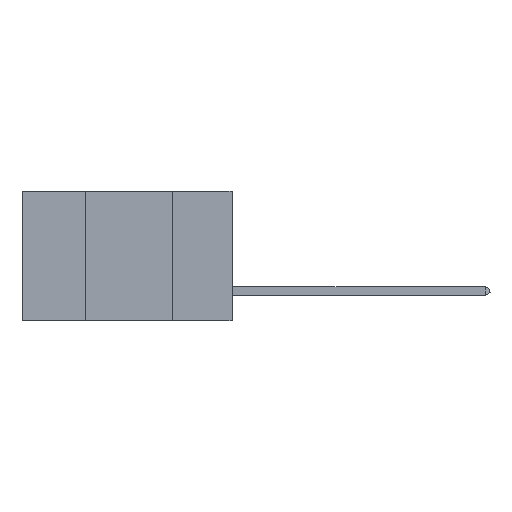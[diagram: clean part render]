
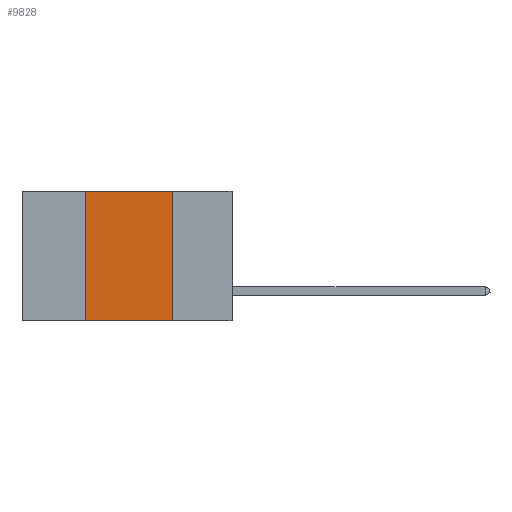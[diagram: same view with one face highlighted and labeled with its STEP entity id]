
A CAD part, left-side view. The second image highlights one B-rep face of the part: STEP entity #9828.
In plain terms, the highlighted planar face has unit normal (-1, 0, 0).
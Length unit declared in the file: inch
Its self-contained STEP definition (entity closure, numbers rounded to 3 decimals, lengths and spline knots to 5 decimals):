
#146 = CARTESIAN_POINT ( 'NONE',  ( 0., 0.42, -0.37 ) ) ;
#923 = CARTESIAN_POINT ( 'NONE',  ( 0., 0.17, 0. ) ) ;
#2415 = EDGE_CURVE ( 'NONE', #5832, #20994, #16432, .T. ) ;
#2769 = ORIENTED_EDGE ( 'NONE', *, *, #3607, .F. ) ;
#3252 = CARTESIAN_POINT ( 'NONE',  ( 0., 0.6, -0.37 ) ) ;
#3427 = CARTESIAN_POINT ( 'NONE',  ( 0., 0.6, 0. ) ) ;
#3607 = EDGE_CURVE ( 'NONE', #13845, #20994, #19619, .T. ) ;
#5685 = VECTOR ( 'NONE', #18300, 39.37008 ) ;
#5832 = VERTEX_POINT ( 'NONE', #146 ) ;
#5968 = VECTOR ( 'NONE', #15742, 39.37008 ) ;
#6342 = EDGE_CURVE ( 'NONE', #8032, #13845, #15232, .T. ) ;
#6881 = DIRECTION ( 'NONE',  ( 0., 0., -1. ) ) ;
#7025 = DIRECTION ( 'NONE',  ( 0., 0., 1. ) ) ;
#8032 = VERTEX_POINT ( 'NONE', #15239 ) ;
#8890 = EDGE_CURVE ( 'NONE', #5832, #8032, #10215, .T. ) ;
#8909 = CARTESIAN_POINT ( 'NONE',  ( 0., 0.17, -0.37 ) ) ;
#8925 = PLANE ( 'NONE',  #9853 ) ;
#9828 = ADVANCED_FACE ( 'NONE', ( #15352 ), #8925, .F. ) ;
#9853 = AXIS2_PLACEMENT_3D ( 'NONE', #3427, #18009, #6881 ) ;
#10215 = LINE ( 'NONE', #23651, #16572 ) ;
#12585 = VECTOR ( 'NONE', #15078, 39.37008 ) ;
#12643 = CARTESIAN_POINT ( 'NONE',  ( 0., 0.6, 0. ) ) ;
#12980 = ORIENTED_EDGE ( 'NONE', *, *, #8890, .F. ) ;
#13845 = VERTEX_POINT ( 'NONE', #923 ) ;
#15078 = DIRECTION ( 'NONE',  ( 0., 0., -1. ) ) ;
#15232 = LINE ( 'NONE', #12643, #5685 ) ;
#15239 = CARTESIAN_POINT ( 'NONE',  ( 0., 0.42, 0. ) ) ;
#15352 = FACE_OUTER_BOUND ( 'NONE', #22428, .T. ) ;
#15742 = DIRECTION ( 'NONE',  ( 0., -1., 0. ) ) ;
#16432 = LINE ( 'NONE', #3252, #5968 ) ;
#16572 = VECTOR ( 'NONE', #7025, 39.37008 ) ;
#18009 = DIRECTION ( 'NONE',  ( 1., 0., 0. ) ) ;
#18300 = DIRECTION ( 'NONE',  ( 0., -1., 0. ) ) ;
#18707 = CARTESIAN_POINT ( 'NONE',  ( 0., 0.17, 0. ) ) ;
#19619 = LINE ( 'NONE', #18707, #12585 ) ;
#19766 = ORIENTED_EDGE ( 'NONE', *, *, #2415, .T. ) ;
#20994 = VERTEX_POINT ( 'NONE', #8909 ) ;
#21237 = ORIENTED_EDGE ( 'NONE', *, *, #6342, .F. ) ;
#22428 = EDGE_LOOP ( 'NONE', ( #2769, #21237, #12980, #19766 ) ) ;
#23651 = CARTESIAN_POINT ( 'NONE',  ( 0., 0.42, 0. ) ) ;
